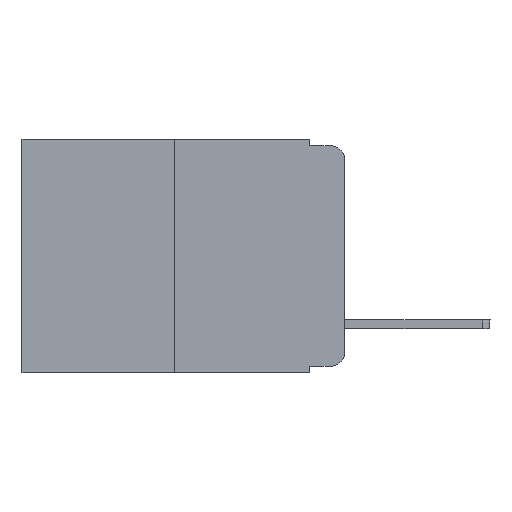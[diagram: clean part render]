
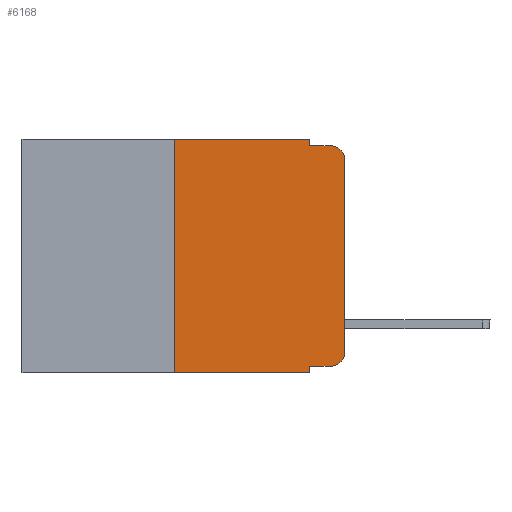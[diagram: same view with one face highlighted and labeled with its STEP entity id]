
A CAD part, left-side view. The second image highlights one B-rep face of the part: STEP entity #6168.
In plain terms, the highlighted planar face has unit normal (-1, 0, 0).
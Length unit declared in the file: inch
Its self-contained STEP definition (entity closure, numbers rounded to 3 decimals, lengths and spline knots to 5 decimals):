
#290 = EDGE_LOOP ( 'NONE', ( #4417, #4964, #2161, #3627, #3743, #9188, #9663, #1559, #8892, #8961 ) ) ;
#395 = VECTOR ( 'NONE', #7269, 39.37008 ) ;
#498 = DIRECTION ( 'NONE',  ( 0., 0., -1. ) ) ;
#580 = EDGE_CURVE ( 'NONE', #10105, #4993, #8134, .T. ) ;
#620 = CARTESIAN_POINT ( 'NONE',  ( 0., 0.25, 0. ) ) ;
#1121 = VECTOR ( 'NONE', #7571, 39.37008 ) ;
#1203 = CARTESIAN_POINT ( 'NONE',  ( 0., 0.051, -0.01 ) ) ;
#1476 = FACE_OUTER_BOUND ( 'NONE', #290, .T. ) ;
#1489 = CARTESIAN_POINT ( 'NONE',  ( 0., 0.02, -0.333 ) ) ;
#1503 = VERTEX_POINT ( 'NONE', #1659 ) ;
#1559 = ORIENTED_EDGE ( 'NONE', *, *, #8686, .F. ) ;
#1570 = CARTESIAN_POINT ( 'NONE',  ( 0., 0.25, -0.343 ) ) ;
#1659 = CARTESIAN_POINT ( 'NONE',  ( 0., 0., -0.313 ) ) ;
#1687 = LINE ( 'NONE', #7623, #5416 ) ;
#2057 = LINE ( 'NONE', #9832, #395 ) ;
#2161 = ORIENTED_EDGE ( 'NONE', *, *, #2832, .F. ) ;
#2174 = CARTESIAN_POINT ( 'NONE',  ( 0., 0.051, 0. ) ) ;
#2191 = VECTOR ( 'NONE', #5209, 39.37008 ) ;
#2212 = DIRECTION ( 'NONE',  ( 0., -1., 0. ) ) ;
#2361 = CARTESIAN_POINT ( 'NONE',  ( 0., 0., -0.03 ) ) ;
#2455 = CARTESIAN_POINT ( 'NONE',  ( 0., 0.051, -0.343 ) ) ;
#2761 = DIRECTION ( 'NONE',  ( 0., 0., -1. ) ) ;
#2832 = EDGE_CURVE ( 'NONE', #4764, #5338, #10249, .T. ) ;
#2888 = EDGE_CURVE ( 'NONE', #10105, #3140, #1687, .T. ) ;
#2973 = CARTESIAN_POINT ( 'NONE',  ( 0., 0.02, -0.313 ) ) ;
#3140 = VERTEX_POINT ( 'NONE', #620 ) ;
#3558 = EDGE_CURVE ( 'NONE', #3140, #6926, #2057, .T. ) ;
#3610 = DIRECTION ( 'NONE',  ( -1., 0., 0. ) ) ;
#3627 = ORIENTED_EDGE ( 'NONE', *, *, #4122, .F. ) ;
#3743 = ORIENTED_EDGE ( 'NONE', *, *, #3558, .F. ) ;
#3921 = VECTOR ( 'NONE', #498, 39.37008 ) ;
#4122 = EDGE_CURVE ( 'NONE', #6926, #4764, #7780, .T. ) ;
#4404 = DIRECTION ( 'NONE',  ( 0., -1., 0. ) ) ;
#4417 = ORIENTED_EDGE ( 'NONE', *, *, #7611, .T. ) ;
#4455 = VECTOR ( 'NONE', #4404, 39.37008 ) ;
#4580 = EDGE_CURVE ( 'NONE', #9238, #8709, #6093, .T. ) ;
#4701 = DIRECTION ( 'NONE',  ( 0., 0., -1. ) ) ;
#4764 = VERTEX_POINT ( 'NONE', #1203 ) ;
#4767 = DIRECTION ( 'NONE',  ( 1., 0., 0. ) ) ;
#4801 = CIRCLE ( 'NONE', #10525, 0.02 ) ;
#4835 = PLANE ( 'NONE',  #5378 ) ;
#4964 = ORIENTED_EDGE ( 'NONE', *, *, #9378, .T. ) ;
#4993 = VERTEX_POINT ( 'NONE', #2455 ) ;
#5209 = DIRECTION ( 'NONE',  ( 0., 0., -1. ) ) ;
#5298 = CARTESIAN_POINT ( 'NONE',  ( 0., 0.051, -0.333 ) ) ;
#5338 = VERTEX_POINT ( 'NONE', #8365 ) ;
#5378 = AXIS2_PLACEMENT_3D ( 'NONE', #10929, #4767, #6690 ) ;
#5416 = VECTOR ( 'NONE', #8560, 39.37008 ) ;
#5517 = AXIS2_PLACEMENT_3D ( 'NONE', #2973, #7178, #4701 ) ;
#5886 = CIRCLE ( 'NONE', #5517, 0.02 ) ;
#6056 = CARTESIAN_POINT ( 'NONE',  ( 0., 0., 0. ) ) ;
#6093 = LINE ( 'NONE', #5298, #4455 ) ;
#6168 = ADVANCED_FACE ( 'NONE', ( #1476 ), #4835, .F. ) ;
#6234 = CARTESIAN_POINT ( 'NONE',  ( 0., 0.02, -0.03 ) ) ;
#6543 = LINE ( 'NONE', #2174, #3921 ) ;
#6690 = DIRECTION ( 'NONE',  ( 0., 0., -1. ) ) ;
#6793 = CARTESIAN_POINT ( 'NONE',  ( 0., 0.051, 0. ) ) ;
#6926 = VERTEX_POINT ( 'NONE', #9672 ) ;
#7178 = DIRECTION ( 'NONE',  ( -1., 0., 0. ) ) ;
#7269 = DIRECTION ( 'NONE',  ( 0., -1., 0. ) ) ;
#7424 = VECTOR ( 'NONE', #2212, 39.37008 ) ;
#7571 = DIRECTION ( 'NONE',  ( 0., -1., 0. ) ) ;
#7611 = EDGE_CURVE ( 'NONE', #1503, #9606, #10046, .T. ) ;
#7623 = CARTESIAN_POINT ( 'NONE',  ( 0., 0.25, 0. ) ) ;
#7780 = LINE ( 'NONE', #6793, #2191 ) ;
#8134 = LINE ( 'NONE', #8917, #7424 ) ;
#8365 = CARTESIAN_POINT ( 'NONE',  ( 0., 0.02, -0.01 ) ) ;
#8366 = VECTOR ( 'NONE', #9512, 39.37008 ) ;
#8560 = DIRECTION ( 'NONE',  ( 0., 0., 1. ) ) ;
#8686 = EDGE_CURVE ( 'NONE', #9238, #4993, #6543, .T. ) ;
#8709 = VERTEX_POINT ( 'NONE', #1489 ) ;
#8892 = ORIENTED_EDGE ( 'NONE', *, *, #4580, .T. ) ;
#8917 = CARTESIAN_POINT ( 'NONE',  ( 0., 0.473, -0.343 ) ) ;
#8961 = ORIENTED_EDGE ( 'NONE', *, *, #9904, .T. ) ;
#9188 = ORIENTED_EDGE ( 'NONE', *, *, #2888, .F. ) ;
#9238 = VERTEX_POINT ( 'NONE', #9362 ) ;
#9362 = CARTESIAN_POINT ( 'NONE',  ( 0., 0.051, -0.333 ) ) ;
#9378 = EDGE_CURVE ( 'NONE', #9606, #5338, #4801, .T. ) ;
#9454 = CARTESIAN_POINT ( 'NONE',  ( 0., 0.051, -0.01 ) ) ;
#9512 = DIRECTION ( 'NONE',  ( 0., 0., 1. ) ) ;
#9606 = VERTEX_POINT ( 'NONE', #2361 ) ;
#9663 = ORIENTED_EDGE ( 'NONE', *, *, #580, .T. ) ;
#9672 = CARTESIAN_POINT ( 'NONE',  ( 0., 0.051, 0. ) ) ;
#9832 = CARTESIAN_POINT ( 'NONE',  ( 0., 0.473, 0. ) ) ;
#9904 = EDGE_CURVE ( 'NONE', #8709, #1503, #5886, .T. ) ;
#10046 = LINE ( 'NONE', #6056, #8366 ) ;
#10105 = VERTEX_POINT ( 'NONE', #1570 ) ;
#10249 = LINE ( 'NONE', #9454, #1121 ) ;
#10525 = AXIS2_PLACEMENT_3D ( 'NONE', #6234, #3610, #2761 ) ;
#10929 = CARTESIAN_POINT ( 'NONE',  ( 0., 0.473, 0. ) ) ;
